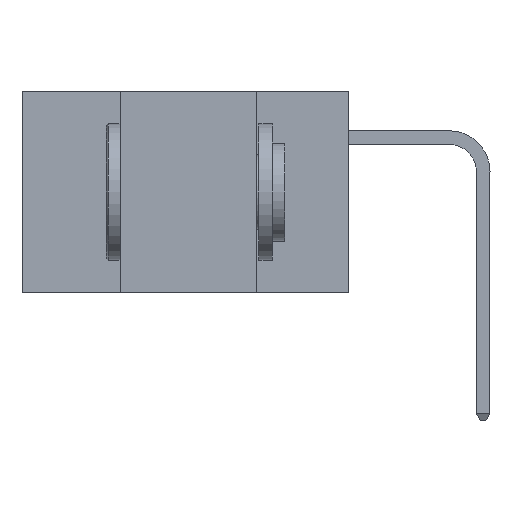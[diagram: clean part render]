
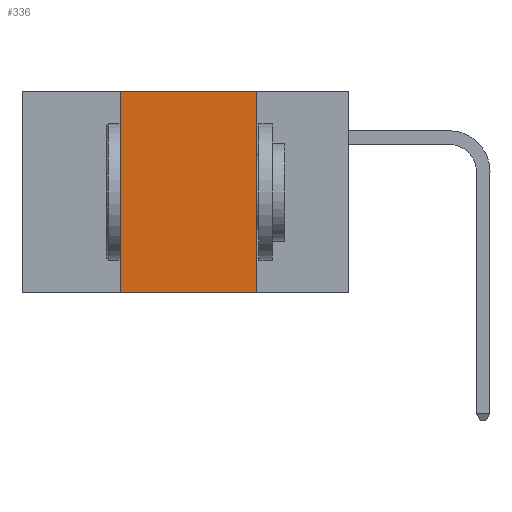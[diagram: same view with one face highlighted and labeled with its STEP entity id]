
A CAD part, left-side view. The second image highlights one B-rep face of the part: STEP entity #336.
In plain terms, the highlighted planar face has unit normal (-1, 0, 0).
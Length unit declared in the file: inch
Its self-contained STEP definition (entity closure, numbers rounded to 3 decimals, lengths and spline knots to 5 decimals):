
#1 = DIRECTION ( 'NONE',  ( 1., 0., 0. ) ) ;
#336 = ADVANCED_FACE ( 'NONE', ( #28797 ), #14183, .F. ) ;
#431 = VECTOR ( 'NONE', #23911, 39.37008 ) ;
#2240 = EDGE_CURVE ( 'NONE', #20222, #15899, #5357, .T. ) ;
#3106 = CARTESIAN_POINT ( 'NONE',  ( 0., 0.42, -0.37 ) ) ;
#5357 = LINE ( 'NONE', #6863, #25331 ) ;
#6678 = ORIENTED_EDGE ( 'NONE', *, *, #2240, .T. ) ;
#6832 = VECTOR ( 'NONE', #17104, 39.37008 ) ;
#6863 = CARTESIAN_POINT ( 'NONE',  ( 0., 0.6, -0.37 ) ) ;
#8846 = EDGE_LOOP ( 'NONE', ( #20938, #22014, #18134, #6678 ) ) ;
#9121 = CARTESIAN_POINT ( 'NONE',  ( 0., 0.17, 0. ) ) ;
#11236 = VECTOR ( 'NONE', #11252, 39.37008 ) ;
#11252 = DIRECTION ( 'NONE',  ( 0., 0., -1. ) ) ;
#11291 = EDGE_CURVE ( 'NONE', #20222, #11482, #14526, .T. ) ;
#11482 = VERTEX_POINT ( 'NONE', #13031 ) ;
#12883 = AXIS2_PLACEMENT_3D ( 'NONE', #26197, #1, #16558 ) ;
#13031 = CARTESIAN_POINT ( 'NONE',  ( 0., 0.42, 0. ) ) ;
#14183 = PLANE ( 'NONE',  #12883 ) ;
#14396 = CARTESIAN_POINT ( 'NONE',  ( 0., 0.42, 0. ) ) ;
#14526 = LINE ( 'NONE', #14396, #431 ) ;
#15374 = LINE ( 'NONE', #26331, #6832 ) ;
#15899 = VERTEX_POINT ( 'NONE', #23140 ) ;
#16558 = DIRECTION ( 'NONE',  ( 0., 0., -1. ) ) ;
#17104 = DIRECTION ( 'NONE',  ( 0., -1., 0. ) ) ;
#17526 = LINE ( 'NONE', #27710, #11236 ) ;
#18134 = ORIENTED_EDGE ( 'NONE', *, *, #11291, .F. ) ;
#19069 = DIRECTION ( 'NONE',  ( 0., -1., 0. ) ) ;
#20222 = VERTEX_POINT ( 'NONE', #3106 ) ;
#20938 = ORIENTED_EDGE ( 'NONE', *, *, #22584, .F. ) ;
#21461 = EDGE_CURVE ( 'NONE', #11482, #26645, #15374, .T. ) ;
#22014 = ORIENTED_EDGE ( 'NONE', *, *, #21461, .F. ) ;
#22584 = EDGE_CURVE ( 'NONE', #26645, #15899, #17526, .T. ) ;
#23140 = CARTESIAN_POINT ( 'NONE',  ( 0., 0.17, -0.37 ) ) ;
#23911 = DIRECTION ( 'NONE',  ( 0., 0., 1. ) ) ;
#25331 = VECTOR ( 'NONE', #19069, 39.37008 ) ;
#26197 = CARTESIAN_POINT ( 'NONE',  ( 0., 0.6, 0. ) ) ;
#26331 = CARTESIAN_POINT ( 'NONE',  ( 0., 0.6, 0. ) ) ;
#26645 = VERTEX_POINT ( 'NONE', #9121 ) ;
#27710 = CARTESIAN_POINT ( 'NONE',  ( 0., 0.17, 0. ) ) ;
#28797 = FACE_OUTER_BOUND ( 'NONE', #8846, .T. ) ;
